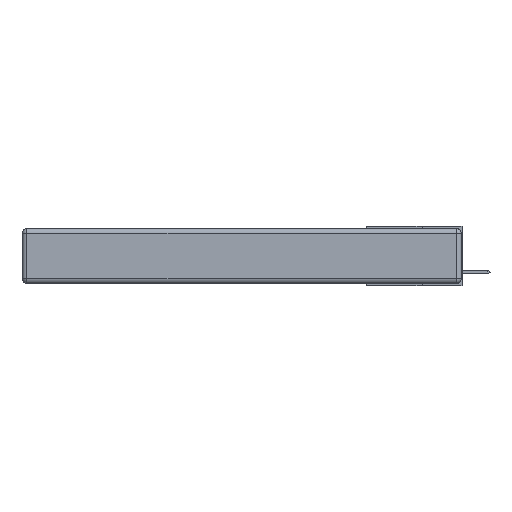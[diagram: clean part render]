
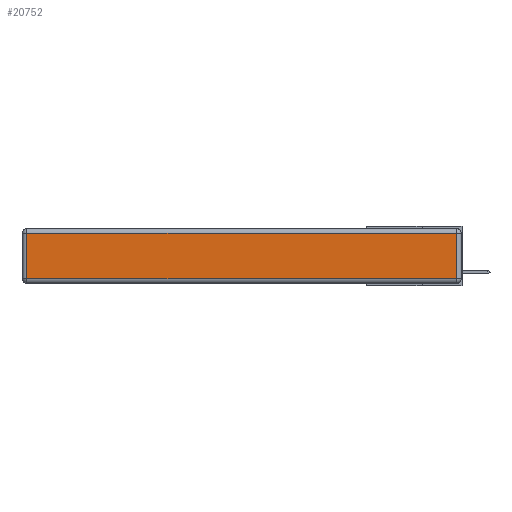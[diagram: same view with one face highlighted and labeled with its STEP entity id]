
A CAD part, left-side view. The second image highlights one B-rep face of the part: STEP entity #20752.
In plain terms, the highlighted planar face has unit normal (-1, 0, 0).
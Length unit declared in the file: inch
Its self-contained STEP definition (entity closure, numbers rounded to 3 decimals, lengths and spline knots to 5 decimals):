
#1045 = EDGE_LOOP ( 'NONE', ( #19491, #4673, #11659, #7316 ) ) ;
#1445 = VERTEX_POINT ( 'NONE', #15788 ) ;
#2398 = VECTOR ( 'NONE', #21034, 39.37008 ) ;
#2578 = DIRECTION ( 'NONE',  ( 0., -1., 0. ) ) ;
#2898 = VECTOR ( 'NONE', #2578, 39.37008 ) ;
#3097 = PLANE ( 'NONE',  #16390 ) ;
#4673 = ORIENTED_EDGE ( 'NONE', *, *, #12909, .T. ) ;
#4971 = LINE ( 'NONE', #6227, #13433 ) ;
#6087 = CARTESIAN_POINT ( 'NONE',  ( 0., 0., -0.313 ) ) ;
#6227 = CARTESIAN_POINT ( 'NONE',  ( 0., 2.72, -0.343 ) ) ;
#7316 = ORIENTED_EDGE ( 'NONE', *, *, #13594, .T. ) ;
#9427 = CARTESIAN_POINT ( 'NONE',  ( 0., 0.03, -0.313 ) ) ;
#9601 = CARTESIAN_POINT ( 'NONE',  ( 0., 0., -0.343 ) ) ;
#9887 = VERTEX_POINT ( 'NONE', #9427 ) ;
#11365 = DIRECTION ( 'NONE',  ( 0., 0., 1. ) ) ;
#11637 = CARTESIAN_POINT ( 'NONE',  ( 0., 0.03, -0.03 ) ) ;
#11659 = ORIENTED_EDGE ( 'NONE', *, *, #21331, .T. ) ;
#12909 = EDGE_CURVE ( 'NONE', #9887, #14729, #16368, .T. ) ;
#12925 = LINE ( 'NONE', #6087, #2898 ) ;
#13433 = VECTOR ( 'NONE', #21529, 39.37008 ) ;
#13594 = EDGE_CURVE ( 'NONE', #1445, #16910, #4971, .T. ) ;
#13798 = DIRECTION ( 'NONE',  ( 0., 1., 0. ) ) ;
#14729 = VERTEX_POINT ( 'NONE', #11637 ) ;
#15258 = FACE_OUTER_BOUND ( 'NONE', #1045, .T. ) ;
#15788 = CARTESIAN_POINT ( 'NONE',  ( 0., 2.72, -0.03 ) ) ;
#16214 = DIRECTION ( 'NONE',  ( -1., 0., 0. ) ) ;
#16368 = LINE ( 'NONE', #19424, #2398 ) ;
#16390 = AXIS2_PLACEMENT_3D ( 'NONE', #9601, #16214, #11365 ) ;
#16910 = VERTEX_POINT ( 'NONE', #16961 ) ;
#16961 = CARTESIAN_POINT ( 'NONE',  ( 0., 2.72, -0.313 ) ) ;
#18773 = CARTESIAN_POINT ( 'NONE',  ( 0., 2.75, -0.03 ) ) ;
#19377 = LINE ( 'NONE', #18773, #20435 ) ;
#19424 = CARTESIAN_POINT ( 'NONE',  ( 0., 0.03, -0.343 ) ) ;
#19491 = ORIENTED_EDGE ( 'NONE', *, *, #20547, .T. ) ;
#20435 = VECTOR ( 'NONE', #13798, 39.37008 ) ;
#20547 = EDGE_CURVE ( 'NONE', #16910, #9887, #12925, .T. ) ;
#20752 = ADVANCED_FACE ( 'NONE', ( #15258 ), #3097, .T. ) ;
#21034 = DIRECTION ( 'NONE',  ( 0., 0., 1. ) ) ;
#21331 = EDGE_CURVE ( 'NONE', #14729, #1445, #19377, .T. ) ;
#21529 = DIRECTION ( 'NONE',  ( 0., 0., -1. ) ) ;
